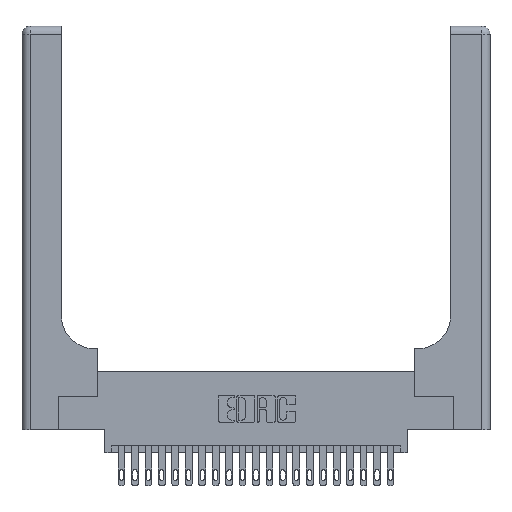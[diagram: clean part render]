
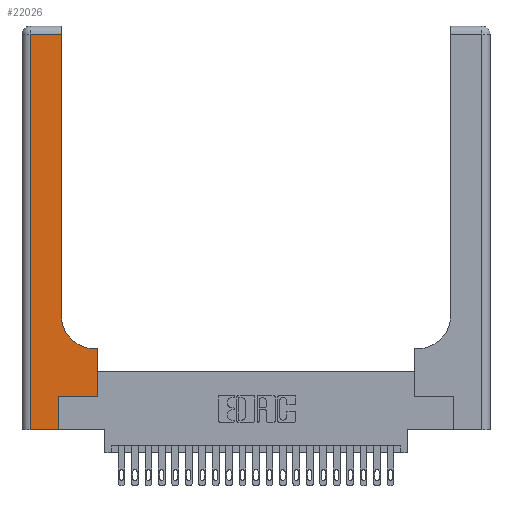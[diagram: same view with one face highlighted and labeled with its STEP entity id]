
A CAD part, top view. The second image highlights one B-rep face of the part: STEP entity #22026.
In plain terms, the highlighted planar face has unit normal (0, 0, 1).
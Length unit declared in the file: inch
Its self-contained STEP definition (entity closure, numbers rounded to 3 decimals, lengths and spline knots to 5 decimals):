
#485 = EDGE_CURVE ( 'NONE', #9465, #11780, #17139, .T. ) ;
#590 = EDGE_CURVE ( 'NONE', #11780, #9105, #23356, .T. ) ;
#1032 = CARTESIAN_POINT ( 'NONE',  ( 0.269, 0., 0.37 ) ) ;
#1045 = ORIENTED_EDGE ( 'NONE', *, *, #15536, .T. ) ;
#1182 = EDGE_CURVE ( 'NONE', #18364, #24567, #12096, .T. ) ;
#1205 = DIRECTION ( 'NONE',  ( 0., -1., 0. ) ) ;
#1797 = VERTEX_POINT ( 'NONE', #10662 ) ;
#2594 = DIRECTION ( 'NONE',  ( 1., 0., 0. ) ) ;
#2618 = CARTESIAN_POINT ( 'NONE',  ( 0.06, 3., 0.37 ) ) ;
#3463 = VECTOR ( 'NONE', #20614, 39.37008 ) ;
#3866 = FACE_OUTER_BOUND ( 'NONE', #11697, .T. ) ;
#3935 = VECTOR ( 'NONE', #4057, 39.37008 ) ;
#4057 = DIRECTION ( 'NONE',  ( 1., 0., 0. ) ) ;
#4588 = EDGE_CURVE ( 'NONE', #9105, #1797, #20068, .T. ) ;
#5391 = CARTESIAN_POINT ( 'NONE',  ( 0.06, 2.94, 0.37 ) ) ;
#5722 = VECTOR ( 'NONE', #19498, 39.37008 ) ;
#6144 = VECTOR ( 'NONE', #1205, 39.37008 ) ;
#6283 = DIRECTION ( 'NONE',  ( 1., 0., 0. ) ) ;
#6451 = CARTESIAN_POINT ( 'NONE',  ( 0., 3., 0.37 ) ) ;
#6549 = CARTESIAN_POINT ( 'NONE',  ( 0.5585, 0.25, 0.37 ) ) ;
#6691 = EDGE_CURVE ( 'NONE', #24090, #7208, #24082, .T. ) ;
#6768 = PLANE ( 'NONE',  #16445 ) ;
#7208 = VERTEX_POINT ( 'NONE', #1032 ) ;
#7521 = ORIENTED_EDGE ( 'NONE', *, *, #590, .T. ) ;
#8646 = EDGE_CURVE ( 'NONE', #24567, #24090, #11210, .T. ) ;
#8688 = DIRECTION ( 'NONE',  ( -1., 0., 0. ) ) ;
#9105 = VERTEX_POINT ( 'NONE', #10060 ) ;
#9465 = VERTEX_POINT ( 'NONE', #10030 ) ;
#9736 = CARTESIAN_POINT ( 'NONE',  ( 0.2915, 2.94, 0.37 ) ) ;
#9980 = VECTOR ( 'NONE', #21364, 39.37008 ) ;
#10030 = CARTESIAN_POINT ( 'NONE',  ( 0.269, 0.25, 0.37 ) ) ;
#10060 = CARTESIAN_POINT ( 'NONE',  ( 0.5585, 0.6, 0.37 ) ) ;
#10354 = DIRECTION ( 'NONE',  ( 0., 0., -1. ) ) ;
#10492 = CARTESIAN_POINT ( 'NONE',  ( 0.2915, 0.85, 0.37 ) ) ;
#10618 = ORIENTED_EDGE ( 'NONE', *, *, #13623, .T. ) ;
#10662 = CARTESIAN_POINT ( 'NONE',  ( 0.5415, 0.6, 0.37 ) ) ;
#11082 = LINE ( 'NONE', #17362, #5722 ) ;
#11210 = LINE ( 'NONE', #2618, #6144 ) ;
#11477 = CARTESIAN_POINT ( 'NONE',  ( 0., 0., 0.37 ) ) ;
#11646 = CARTESIAN_POINT ( 'NONE',  ( 0.269, 0.25, 0.37 ) ) ;
#11697 = EDGE_LOOP ( 'NONE', ( #10618, #18472, #11941, #19381, #1045, #13673, #7521, #15343, #23922 ) ) ;
#11740 = CARTESIAN_POINT ( 'NONE',  ( 0.5585, 0.25, 0.37 ) ) ;
#11780 = VERTEX_POINT ( 'NONE', #11740 ) ;
#11941 = ORIENTED_EDGE ( 'NONE', *, *, #8646, .T. ) ;
#12096 = LINE ( 'NONE', #18687, #3463 ) ;
#13083 = CIRCLE ( 'NONE', #22360, 0.25 ) ;
#13294 = VECTOR ( 'NONE', #14335, 39.37008 ) ;
#13623 = EDGE_CURVE ( 'NONE', #18481, #18364, #11082, .T. ) ;
#13673 = ORIENTED_EDGE ( 'NONE', *, *, #485, .T. ) ;
#14335 = DIRECTION ( 'NONE',  ( 0., 1., 0. ) ) ;
#15340 = LINE ( 'NONE', #20745, #22123 ) ;
#15343 = ORIENTED_EDGE ( 'NONE', *, *, #4588, .T. ) ;
#15536 = EDGE_CURVE ( 'NONE', #7208, #9465, #15340, .T. ) ;
#16276 = EDGE_CURVE ( 'NONE', #1797, #18481, #13083, .T. ) ;
#16445 = AXIS2_PLACEMENT_3D ( 'NONE', #6451, #10354, #8688 ) ;
#17050 = CARTESIAN_POINT ( 'NONE',  ( 0.2915, 0.6, 0.37 ) ) ;
#17113 = DIRECTION ( 'NONE',  ( 0., 1., 0. ) ) ;
#17139 = LINE ( 'NONE', #11646, #18314 ) ;
#17362 = CARTESIAN_POINT ( 'NONE',  ( 0.2915, 3., 0.37 ) ) ;
#18314 = VECTOR ( 'NONE', #2594, 39.37008 ) ;
#18364 = VERTEX_POINT ( 'NONE', #9736 ) ;
#18472 = ORIENTED_EDGE ( 'NONE', *, *, #1182, .T. ) ;
#18477 = CARTESIAN_POINT ( 'NONE',  ( 0.06, 0., 0.37 ) ) ;
#18481 = VERTEX_POINT ( 'NONE', #10492 ) ;
#18687 = CARTESIAN_POINT ( 'NONE',  ( 0., 2.94, 0.37 ) ) ;
#19381 = ORIENTED_EDGE ( 'NONE', *, *, #6691, .T. ) ;
#19498 = DIRECTION ( 'NONE',  ( 0., 1., 0. ) ) ;
#20068 = LINE ( 'NONE', #17050, #9980 ) ;
#20614 = DIRECTION ( 'NONE',  ( -1., 0., 0. ) ) ;
#20745 = CARTESIAN_POINT ( 'NONE',  ( 0.269, 0., 0.37 ) ) ;
#21364 = DIRECTION ( 'NONE',  ( -1., 0., 0. ) ) ;
#21443 = CARTESIAN_POINT ( 'NONE',  ( 0.5415, 0.85, 0.37 ) ) ;
#22026 = ADVANCED_FACE ( 'NONE', ( #3866 ), #6768, .F. ) ;
#22123 = VECTOR ( 'NONE', #17113, 39.37008 ) ;
#22360 = AXIS2_PLACEMENT_3D ( 'NONE', #21443, #23088, #6283 ) ;
#23088 = DIRECTION ( 'NONE',  ( 0., 0., -1. ) ) ;
#23356 = LINE ( 'NONE', #6549, #13294 ) ;
#23922 = ORIENTED_EDGE ( 'NONE', *, *, #16276, .T. ) ;
#24082 = LINE ( 'NONE', #11477, #3935 ) ;
#24090 = VERTEX_POINT ( 'NONE', #18477 ) ;
#24567 = VERTEX_POINT ( 'NONE', #5391 ) ;
